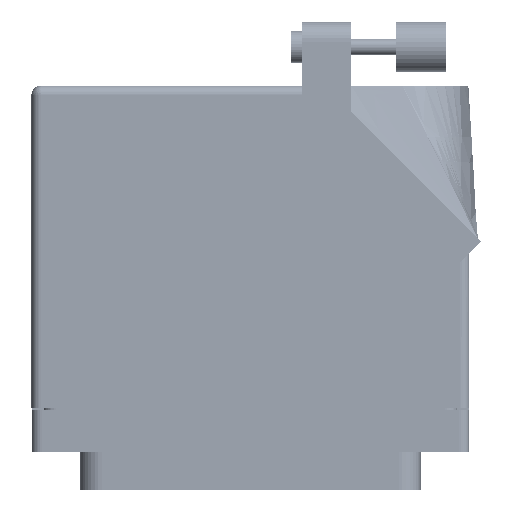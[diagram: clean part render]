
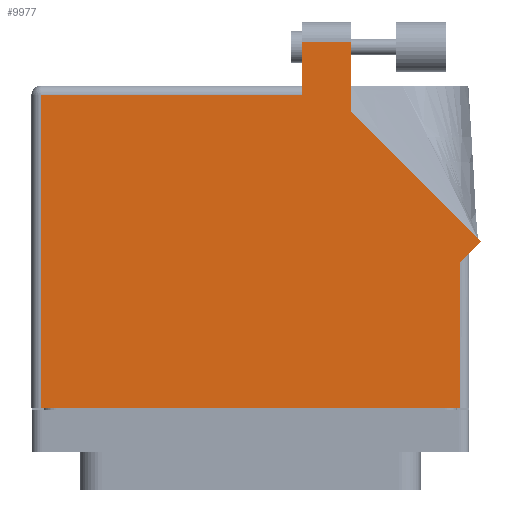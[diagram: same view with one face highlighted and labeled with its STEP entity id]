
A CAD part, front view. The second image highlights one B-rep face of the part: STEP entity #9977.
In plain terms, the highlighted face is planar.
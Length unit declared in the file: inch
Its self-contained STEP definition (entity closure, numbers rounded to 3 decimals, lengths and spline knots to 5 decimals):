
#1218 = LINE ( 'NONE', #40795, #45428 ) ;
#2611 = CARTESIAN_POINT ( 'NONE',  ( 1.3155, -0.1, 0.765 ) ) ;
#3185 = VERTEX_POINT ( 'NONE', #11108 ) ;
#6149 = ORIENTED_EDGE ( 'NONE', *, *, #38716, .T. ) ;
#7237 = ORIENTED_EDGE ( 'NONE', *, *, #49242, .T. ) ;
#8027 = DIRECTION ( 'NONE',  ( 0., 0., -1. ) ) ;
#8433 = AXIS2_PLACEMENT_3D ( 'NONE', #14403, #8027, #42409 ) ;
#9530 = VECTOR ( 'NONE', #37310, 39.37008 ) ;
#9977 = ADVANCED_FACE ( 'NONE', ( #74745 ), #62846, .F. ) ;
#10464 = LINE ( 'NONE', #10473, #9530 ) ;
#10473 = CARTESIAN_POINT ( 'NONE',  ( -1.3155, -0.1, 0.765 ) ) ;
#11108 = CARTESIAN_POINT ( 'NONE',  ( 0.3275, 2.205, 0.765 ) ) ;
#11132 = EDGE_CURVE ( 'NONE', #85118, #70079, #1218, .T. ) ;
#11600 = CARTESIAN_POINT ( 'NONE',  ( 0.6345, 2.205, 0.765 ) ) ;
#12279 = VECTOR ( 'NONE', #86275, 39.37008 ) ;
#14403 = CARTESIAN_POINT ( 'NONE',  ( -1.3775, 1.93, 0.765 ) ) ;
#17220 = ORIENTED_EDGE ( 'NONE', *, *, #59003, .T. ) ;
#17676 = VECTOR ( 'NONE', #43236, 39.37008 ) ;
#18552 = VECTOR ( 'NONE', #25427, 39.37008 ) ;
#19235 = EDGE_CURVE ( 'NONE', #24690, #41895, #71009, .T. ) ;
#19772 = DIRECTION ( 'NONE',  ( 0., 1., 0. ) ) ;
#20252 = DIRECTION ( 'NONE',  ( -0.707, 0.707, 0. ) ) ;
#21166 = VECTOR ( 'NONE', #28813, 39.37008 ) ;
#21751 = ORIENTED_EDGE ( 'NONE', *, *, #41989, .T. ) ;
#22013 = LINE ( 'NONE', #85140, #17676 ) ;
#22769 = CARTESIAN_POINT ( 'NONE',  ( 1.3155, 0.818, 0.765 ) ) ;
#24690 = VERTEX_POINT ( 'NONE', #2611 ) ;
#25427 = DIRECTION ( 'NONE',  ( -1., 0., 0. ) ) ;
#26741 = CARTESIAN_POINT ( 'NONE',  ( 0.3275, 1.868, 0.765 ) ) ;
#28285 = LINE ( 'NONE', #80547, #18552 ) ;
#28813 = DIRECTION ( 'NONE',  ( -1., 0., 0. ) ) ;
#31207 = EDGE_CURVE ( 'NONE', #45339, #80331, #63109, .T. ) ;
#31480 = EDGE_LOOP ( 'NONE', ( #50942, #17220, #7237, #75518, #6149, #51740, #36758, #21751, #67342 ) ) ;
#33780 = CARTESIAN_POINT ( 'NONE',  ( 1.44821, 0.95071, 0.765 ) ) ;
#36758 = ORIENTED_EDGE ( 'NONE', *, *, #19235, .T. ) ;
#37310 = DIRECTION ( 'NONE',  ( 0., -1., 0. ) ) ;
#38716 = EDGE_CURVE ( 'NONE', #80331, #83843, #10464, .T. ) ;
#40795 = CARTESIAN_POINT ( 'NONE',  ( 0.6345, 1.76442, 0.765 ) ) ;
#41895 = VERTEX_POINT ( 'NONE', #22769 ) ;
#41989 = EDGE_CURVE ( 'NONE', #41895, #82957, #22013, .T. ) ;
#42409 = DIRECTION ( 'NONE',  ( -1., 0., 0. ) ) ;
#43236 = DIRECTION ( 'NONE',  ( 0.707, 0.707, 0. ) ) ;
#45339 = VERTEX_POINT ( 'NONE', #26741 ) ;
#45428 = VECTOR ( 'NONE', #19772, 39.37008 ) ;
#49242 = EDGE_CURVE ( 'NONE', #3185, #45339, #80107, .T. ) ;
#50942 = ORIENTED_EDGE ( 'NONE', *, *, #11132, .T. ) ;
#51086 = DIRECTION ( 'NONE',  ( 0., 1., 0. ) ) ;
#51740 = ORIENTED_EDGE ( 'NONE', *, *, #72360, .T. ) ;
#53257 = CARTESIAN_POINT ( 'NONE',  ( 0.6345, 1.76442, 0.765 ) ) ;
#54235 = DIRECTION ( 'NONE',  ( 0., -1., 0. ) ) ;
#54297 = LINE ( 'NONE', #78700, #12279 ) ;
#56516 = CARTESIAN_POINT ( 'NONE',  ( -1.3775, 1.868, 0.765 ) ) ;
#59003 = EDGE_CURVE ( 'NONE', #70079, #3185, #28285, .T. ) ;
#60411 = VECTOR ( 'NONE', #20252, 39.37008 ) ;
#62421 = CARTESIAN_POINT ( 'NONE',  ( -1.3155, 1.868, 0.765 ) ) ;
#62846 = PLANE ( 'NONE',  #8433 ) ;
#63109 = LINE ( 'NONE', #56516, #21166 ) ;
#65589 = CARTESIAN_POINT ( 'NONE',  ( 1.44821, 0.95071, 0.765 ) ) ;
#66921 = LINE ( 'NONE', #33780, #60411 ) ;
#67342 = ORIENTED_EDGE ( 'NONE', *, *, #69610, .T. ) ;
#69610 = EDGE_CURVE ( 'NONE', #82957, #85118, #66921, .T. ) ;
#70079 = VERTEX_POINT ( 'NONE', #11600 ) ;
#71009 = LINE ( 'NONE', #85799, #86199 ) ;
#71420 = VECTOR ( 'NONE', #54235, 39.37008 ) ;
#72360 = EDGE_CURVE ( 'NONE', #83843, #24690, #54297, .T. ) ;
#74745 = FACE_OUTER_BOUND ( 'NONE', #31480, .T. ) ;
#75518 = ORIENTED_EDGE ( 'NONE', *, *, #31207, .T. ) ;
#78700 = CARTESIAN_POINT ( 'NONE',  ( -1.3775, -0.1, 0.765 ) ) ;
#80107 = LINE ( 'NONE', #81677, #71420 ) ;
#80331 = VERTEX_POINT ( 'NONE', #62421 ) ;
#80547 = CARTESIAN_POINT ( 'NONE',  ( 0.3275, 2.205, 0.765 ) ) ;
#81426 = CARTESIAN_POINT ( 'NONE',  ( -1.3155, -0.1, 0.765 ) ) ;
#81677 = CARTESIAN_POINT ( 'NONE',  ( 0.3275, 1.93, 0.765 ) ) ;
#82957 = VERTEX_POINT ( 'NONE', #65589 ) ;
#83843 = VERTEX_POINT ( 'NONE', #81426 ) ;
#85118 = VERTEX_POINT ( 'NONE', #53257 ) ;
#85140 = CARTESIAN_POINT ( 'NONE',  ( 1.3775, 0.88, 0.765 ) ) ;
#85799 = CARTESIAN_POINT ( 'NONE',  ( 1.3155, 0.88, 0.765 ) ) ;
#86199 = VECTOR ( 'NONE', #51086, 39.37008 ) ;
#86275 = DIRECTION ( 'NONE',  ( 1., 0., 0. ) ) ;
